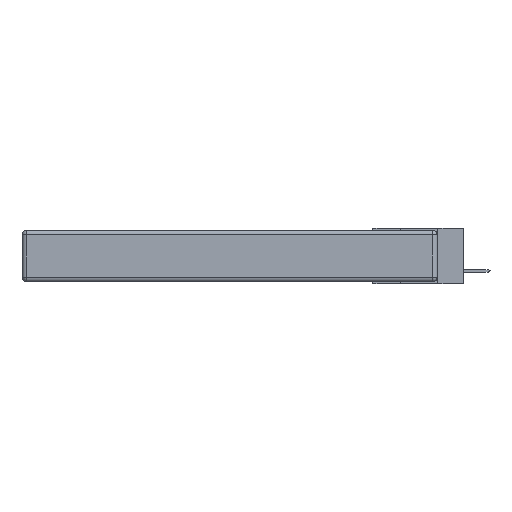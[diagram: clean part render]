
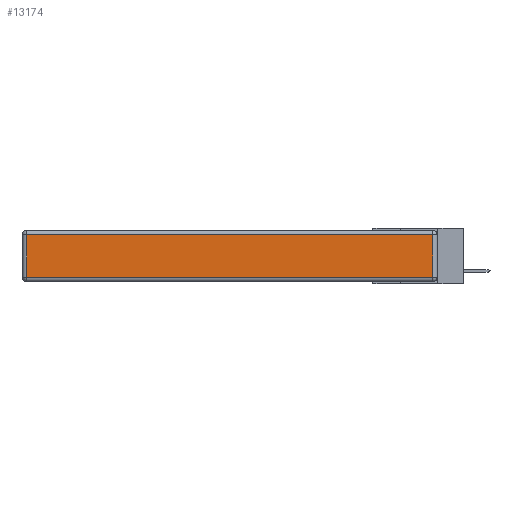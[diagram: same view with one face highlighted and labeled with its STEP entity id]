
A CAD part, left-side view. The second image highlights one B-rep face of the part: STEP entity #13174.
In plain terms, the highlighted planar face has unit normal (-1, 0, 0).
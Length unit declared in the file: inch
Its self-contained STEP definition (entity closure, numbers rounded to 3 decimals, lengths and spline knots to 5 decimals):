
#339 = CARTESIAN_POINT ( 'NONE',  ( 0., 0., -0.313 ) ) ;
#592 = LINE ( 'NONE', #13349, #8366 ) ;
#1389 = VERTEX_POINT ( 'NONE', #8001 ) ;
#4240 = ORIENTED_EDGE ( 'NONE', *, *, #17170, .T. ) ;
#4721 = EDGE_CURVE ( 'NONE', #19700, #13806, #17848, .T. ) ;
#5756 = EDGE_CURVE ( 'NONE', #13806, #1389, #592, .T. ) ;
#5788 = VERTEX_POINT ( 'NONE', #14967 ) ;
#6786 = FACE_OUTER_BOUND ( 'NONE', #15277, .T. ) ;
#6885 = CARTESIAN_POINT ( 'NONE',  ( 0., 0.03, -0.03 ) ) ;
#7092 = CARTESIAN_POINT ( 'NONE',  ( 0., 0.03, -0.343 ) ) ;
#8001 = CARTESIAN_POINT ( 'NONE',  ( 0., 2.72, -0.313 ) ) ;
#8076 = EDGE_CURVE ( 'NONE', #5788, #19700, #13854, .T. ) ;
#8366 = VECTOR ( 'NONE', #11922, 39.37008 ) ;
#8430 = DIRECTION ( 'NONE',  ( 0., 0., 1. ) ) ;
#9982 = DIRECTION ( 'NONE',  ( 0., 0., 1. ) ) ;
#11922 = DIRECTION ( 'NONE',  ( 0., 0., -1. ) ) ;
#12245 = ORIENTED_EDGE ( 'NONE', *, *, #8076, .T. ) ;
#12724 = VECTOR ( 'NONE', #14044, 39.37008 ) ;
#13049 = CARTESIAN_POINT ( 'NONE',  ( 0., 0., -0.343 ) ) ;
#13174 = ADVANCED_FACE ( 'NONE', ( #6786 ), #15966, .T. ) ;
#13349 = CARTESIAN_POINT ( 'NONE',  ( 0., 2.72, -0.343 ) ) ;
#13806 = VERTEX_POINT ( 'NONE', #14384 ) ;
#13854 = LINE ( 'NONE', #7092, #19888 ) ;
#14044 = DIRECTION ( 'NONE',  ( 0., 1., 0. ) ) ;
#14384 = CARTESIAN_POINT ( 'NONE',  ( 0., 2.72, -0.03 ) ) ;
#14446 = DIRECTION ( 'NONE',  ( 0., -1., 0. ) ) ;
#14967 = CARTESIAN_POINT ( 'NONE',  ( 0., 0.03, -0.313 ) ) ;
#15277 = EDGE_LOOP ( 'NONE', ( #4240, #12245, #17432, #20076 ) ) ;
#15585 = VECTOR ( 'NONE', #14446, 39.37008 ) ;
#15966 = PLANE ( 'NONE',  #19998 ) ;
#17170 = EDGE_CURVE ( 'NONE', #1389, #5788, #18980, .T. ) ;
#17432 = ORIENTED_EDGE ( 'NONE', *, *, #4721, .T. ) ;
#17706 = DIRECTION ( 'NONE',  ( -1., 0., 0. ) ) ;
#17848 = LINE ( 'NONE', #18462, #12724 ) ;
#18462 = CARTESIAN_POINT ( 'NONE',  ( 0., 2.75, -0.03 ) ) ;
#18980 = LINE ( 'NONE', #339, #15585 ) ;
#19700 = VERTEX_POINT ( 'NONE', #6885 ) ;
#19888 = VECTOR ( 'NONE', #8430, 39.37008 ) ;
#19998 = AXIS2_PLACEMENT_3D ( 'NONE', #13049, #17706, #9982 ) ;
#20076 = ORIENTED_EDGE ( 'NONE', *, *, #5756, .T. ) ;
